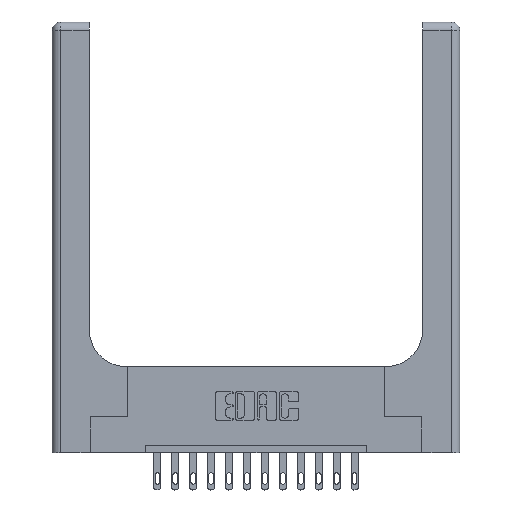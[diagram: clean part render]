
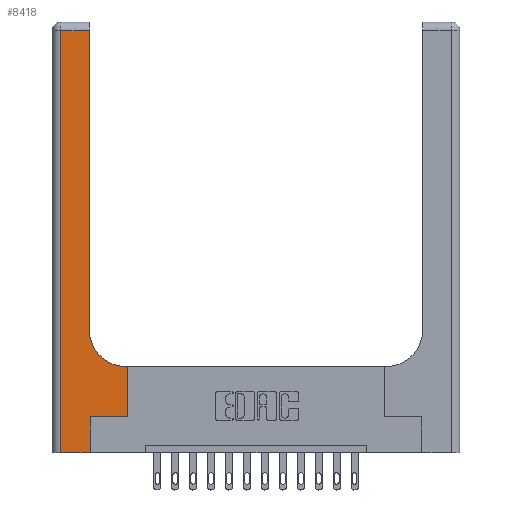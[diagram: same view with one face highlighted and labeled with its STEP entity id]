
A CAD part, top view. The second image highlights one B-rep face of the part: STEP entity #8418.
In plain terms, the highlighted planar face has unit normal (0, 0, 1).
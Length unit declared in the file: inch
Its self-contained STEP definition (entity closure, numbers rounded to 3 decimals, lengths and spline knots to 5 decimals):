
#59 = LINE ( 'NONE', #14531, #3393 ) ;
#64 = LINE ( 'NONE', #11633, #9958 ) ;
#192 = CIRCLE ( 'NONE', #7130, 0.25 ) ;
#214 = LINE ( 'NONE', #5478, #13793 ) ;
#831 = CARTESIAN_POINT ( 'NONE',  ( 0.26, 3., 0.37 ) ) ;
#1485 = CARTESIAN_POINT ( 'NONE',  ( 0.51, 0.85, 0.37 ) ) ;
#1569 = DIRECTION ( 'NONE',  ( 1., 0., 0. ) ) ;
#1647 = DIRECTION ( 'NONE',  ( -1., 0., 0. ) ) ;
#1693 = ORIENTED_EDGE ( 'NONE', *, *, #7068, .T. ) ;
#2185 = PLANE ( 'NONE',  #6891 ) ;
#2361 = CARTESIAN_POINT ( 'NONE',  ( 0.51, 0.6, 0.37 ) ) ;
#2804 = VERTEX_POINT ( 'NONE', #12169 ) ;
#2863 = DIRECTION ( 'NONE',  ( 0., 1., 0. ) ) ;
#3255 = DIRECTION ( 'NONE',  ( 0., 1., 0. ) ) ;
#3393 = VECTOR ( 'NONE', #5323, 39.37008 ) ;
#3495 = DIRECTION ( 'NONE',  ( 0., 1., 0. ) ) ;
#3773 = VERTEX_POINT ( 'NONE', #16171 ) ;
#3883 = VERTEX_POINT ( 'NONE', #14339 ) ;
#4064 = VECTOR ( 'NONE', #2863, 39.37008 ) ;
#4078 = CARTESIAN_POINT ( 'NONE',  ( 0., 2.94, 0.37 ) ) ;
#4369 = DIRECTION ( 'NONE',  ( 1., 0., 0. ) ) ;
#5323 = DIRECTION ( 'NONE',  ( 0., -1., 0. ) ) ;
#5478 = CARTESIAN_POINT ( 'NONE',  ( 0.265, 0.25, 0.37 ) ) ;
#5840 = LINE ( 'NONE', #831, #12098 ) ;
#5851 = VERTEX_POINT ( 'NONE', #10633 ) ;
#5898 = ORIENTED_EDGE ( 'NONE', *, *, #7812, .T. ) ;
#6479 = LINE ( 'NONE', #15945, #4064 ) ;
#6572 = ORIENTED_EDGE ( 'NONE', *, *, #7790, .T. ) ;
#6694 = LINE ( 'NONE', #14285, #16259 ) ;
#6891 = AXIS2_PLACEMENT_3D ( 'NONE', #10125, #7444, #14312 ) ;
#7068 = EDGE_CURVE ( 'NONE', #10142, #14208, #214, .T. ) ;
#7130 = AXIS2_PLACEMENT_3D ( 'NONE', #1485, #11916, #1569 ) ;
#7444 = DIRECTION ( 'NONE',  ( 0., 0., -1. ) ) ;
#7790 = EDGE_CURVE ( 'NONE', #3773, #8449, #6694, .T. ) ;
#7812 = EDGE_CURVE ( 'NONE', #5851, #2804, #64, .T. ) ;
#8136 = VECTOR ( 'NONE', #1647, 39.37008 ) ;
#8418 = ADVANCED_FACE ( 'NONE', ( #9068 ), #2185, .F. ) ;
#8449 = VERTEX_POINT ( 'NONE', #2361 ) ;
#8582 = CARTESIAN_POINT ( 'NONE',  ( 0.265, 0., 0.37 ) ) ;
#8611 = EDGE_CURVE ( 'NONE', #14208, #3773, #6479, .T. ) ;
#9022 = EDGE_LOOP ( 'NONE', ( #9610, #10038, #9335, #5898, #13110, #1693, #11276, #6572, #14761 ) ) ;
#9068 = FACE_OUTER_BOUND ( 'NONE', #9022, .T. ) ;
#9070 = EDGE_CURVE ( 'NONE', #13526, #3883, #5840, .T. ) ;
#9335 = ORIENTED_EDGE ( 'NONE', *, *, #11721, .T. ) ;
#9382 = DIRECTION ( 'NONE',  ( -1., 0., 0. ) ) ;
#9610 = ORIENTED_EDGE ( 'NONE', *, *, #9070, .T. ) ;
#9684 = EDGE_CURVE ( 'NONE', #8449, #13526, #192, .T. ) ;
#9958 = VECTOR ( 'NONE', #16869, 39.37008 ) ;
#10038 = ORIENTED_EDGE ( 'NONE', *, *, #14618, .T. ) ;
#10118 = VERTEX_POINT ( 'NONE', #14382 ) ;
#10125 = CARTESIAN_POINT ( 'NONE',  ( 0., 3., 0.37 ) ) ;
#10142 = VERTEX_POINT ( 'NONE', #13270 ) ;
#10633 = CARTESIAN_POINT ( 'NONE',  ( 0.06, 0., 0.37 ) ) ;
#11276 = ORIENTED_EDGE ( 'NONE', *, *, #8611, .T. ) ;
#11633 = CARTESIAN_POINT ( 'NONE',  ( 0., 0., 0.37 ) ) ;
#11721 = EDGE_CURVE ( 'NONE', #10118, #5851, #59, .T. ) ;
#11916 = DIRECTION ( 'NONE',  ( 0., 0., -1. ) ) ;
#12098 = VECTOR ( 'NONE', #3255, 39.37008 ) ;
#12169 = CARTESIAN_POINT ( 'NONE',  ( 0.265, 0., 0.37 ) ) ;
#12620 = LINE ( 'NONE', #8582, #16921 ) ;
#13110 = ORIENTED_EDGE ( 'NONE', *, *, #16768, .T. ) ;
#13138 = CARTESIAN_POINT ( 'NONE',  ( 0.528, 0.25, 0.37 ) ) ;
#13270 = CARTESIAN_POINT ( 'NONE',  ( 0.265, 0.25, 0.37 ) ) ;
#13526 = VERTEX_POINT ( 'NONE', #16612 ) ;
#13793 = VECTOR ( 'NONE', #4369, 39.37008 ) ;
#14208 = VERTEX_POINT ( 'NONE', #13138 ) ;
#14285 = CARTESIAN_POINT ( 'NONE',  ( 0.26, 0.6, 0.37 ) ) ;
#14312 = DIRECTION ( 'NONE',  ( -1., 0., 0. ) ) ;
#14339 = CARTESIAN_POINT ( 'NONE',  ( 0.26, 2.94, 0.37 ) ) ;
#14382 = CARTESIAN_POINT ( 'NONE',  ( 0.06, 2.94, 0.37 ) ) ;
#14531 = CARTESIAN_POINT ( 'NONE',  ( 0.06, 3., 0.37 ) ) ;
#14618 = EDGE_CURVE ( 'NONE', #3883, #10118, #15861, .T. ) ;
#14761 = ORIENTED_EDGE ( 'NONE', *, *, #9684, .T. ) ;
#15861 = LINE ( 'NONE', #4078, #8136 ) ;
#15945 = CARTESIAN_POINT ( 'NONE',  ( 0.528, 0.25, 0.37 ) ) ;
#16171 = CARTESIAN_POINT ( 'NONE',  ( 0.528, 0.6, 0.37 ) ) ;
#16259 = VECTOR ( 'NONE', #9382, 39.37008 ) ;
#16612 = CARTESIAN_POINT ( 'NONE',  ( 0.26, 0.85, 0.37 ) ) ;
#16768 = EDGE_CURVE ( 'NONE', #2804, #10142, #12620, .T. ) ;
#16869 = DIRECTION ( 'NONE',  ( 1., 0., 0. ) ) ;
#16921 = VECTOR ( 'NONE', #3495, 39.37008 ) ;
